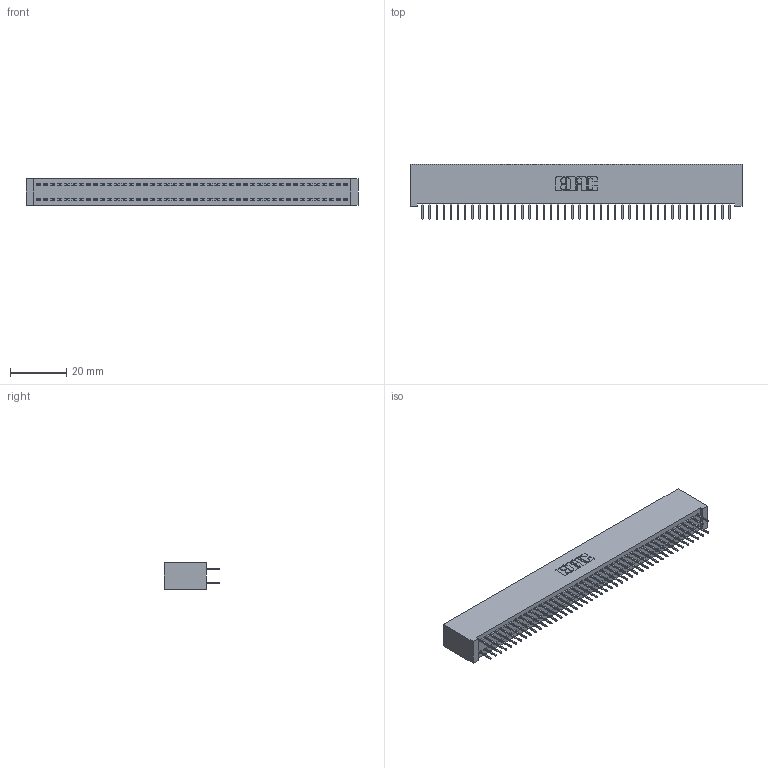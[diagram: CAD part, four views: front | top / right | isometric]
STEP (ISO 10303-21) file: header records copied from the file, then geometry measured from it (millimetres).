
FILE_DESCRIPTION (( 'STEP AP203' ), '1' );
FILE_NAME ('392-088-524-201.STEP', '2019-10-09T16:43:04', ( '' ), ( '' ), 'SwSTEP 2.0', 'SolidWorks 2016', '' );
FILE_SCHEMA (( 'CONFIG_CONTROL_DESIGN' ));
Length unit declared in the file: inch
Products named in the file (3): 342 Part_Lugless; 345-292-001_345-293-124; 392-088-524-201
Assembly tree (89 placements, depth 2):
  392-088-524-201
    342 Part_Lugless
    345-292-001_345-293-124  x88
Bounding box: 118.01 x 19.69 x 9.4 mm (x, y, z)
Volume: 10918.8 mm3; surface area: 17922.3 mm2
Topology: 89 solids, 89 shells, 5030 faces, 14267 edges, 9158 vertices
Faces by surface type: plane 3758, cylinder 1272
Entity records: 27713 total; most frequent: CARTESIAN_POINT 4586, ORIENTED_EDGE 4522, DIRECTION 3909, EDGE_CURVE 2261, LINE 2145, VECTOR 2145, VERTEX_POINT 1502, AXIS2_PLACEMENT_3D 882
